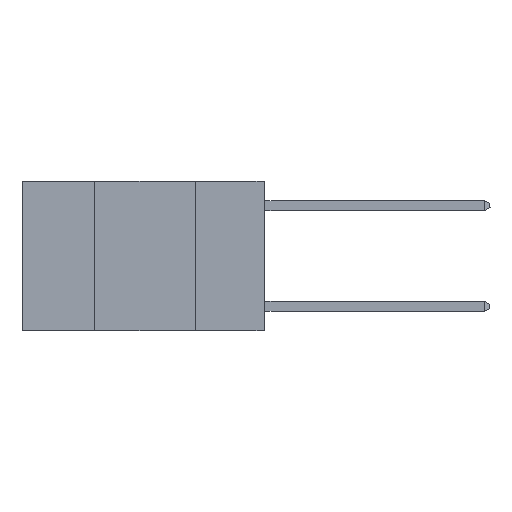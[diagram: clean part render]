
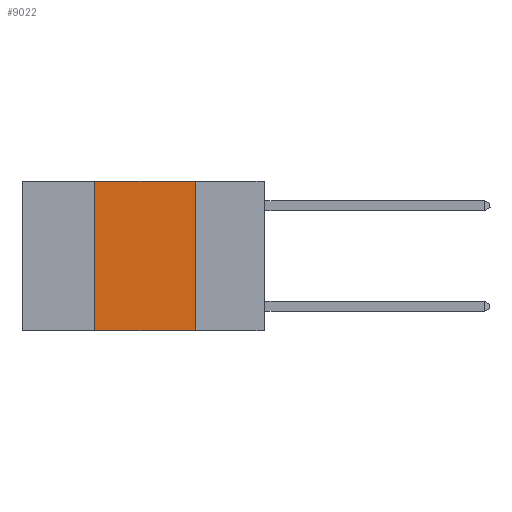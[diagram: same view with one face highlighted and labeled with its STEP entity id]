
A CAD part, left-side view. The second image highlights one B-rep face of the part: STEP entity #9022.
In plain terms, the highlighted planar face has unit normal (-1, 0, 0).
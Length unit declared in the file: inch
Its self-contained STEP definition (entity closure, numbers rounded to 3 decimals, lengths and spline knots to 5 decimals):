
#333 = CARTESIAN_POINT ( 'NONE',  ( 0., 0.17, -0.37 ) ) ;
#363 = ORIENTED_EDGE ( 'NONE', *, *, #10234, .F. ) ;
#574 = EDGE_LOOP ( 'NONE', ( #363, #10213, #7050, #12635 ) ) ;
#619 = VECTOR ( 'NONE', #13344, 39.37008 ) ;
#1965 = DIRECTION ( 'NONE',  ( 0., 0., 1. ) ) ;
#2409 = CARTESIAN_POINT ( 'NONE',  ( 0., 0.6, 0. ) ) ;
#2522 = VERTEX_POINT ( 'NONE', #14680 ) ;
#2852 = EDGE_CURVE ( 'NONE', #5796, #2522, #13362, .T. ) ;
#3385 = DIRECTION ( 'NONE',  ( 0., -1., 0. ) ) ;
#4080 = VECTOR ( 'NONE', #1965, 39.37008 ) ;
#4568 = CARTESIAN_POINT ( 'NONE',  ( 0., 0.42, -0.37 ) ) ;
#4858 = CARTESIAN_POINT ( 'NONE',  ( 0., 0.17, 0. ) ) ;
#5771 = DIRECTION ( 'NONE',  ( 0., -1., 0. ) ) ;
#5796 = VERTEX_POINT ( 'NONE', #4568 ) ;
#7012 = CARTESIAN_POINT ( 'NONE',  ( 0., 0.6, 0. ) ) ;
#7050 = ORIENTED_EDGE ( 'NONE', *, *, #2852, .F. ) ;
#7254 = DIRECTION ( 'NONE',  ( 1., 0., 0. ) ) ;
#7894 = AXIS2_PLACEMENT_3D ( 'NONE', #2409, #7254, #11761 ) ;
#8604 = VECTOR ( 'NONE', #5771, 39.37008 ) ;
#9022 = ADVANCED_FACE ( 'NONE', ( #11317 ), #14506, .F. ) ;
#9568 = VECTOR ( 'NONE', #3385, 39.37008 ) ;
#10213 = ORIENTED_EDGE ( 'NONE', *, *, #10775, .F. ) ;
#10234 = EDGE_CURVE ( 'NONE', #11382, #14653, #13172, .T. ) ;
#10775 = EDGE_CURVE ( 'NONE', #2522, #11382, #12385, .T. ) ;
#11046 = EDGE_CURVE ( 'NONE', #5796, #14653, #11806, .T. ) ;
#11317 = FACE_OUTER_BOUND ( 'NONE', #574, .T. ) ;
#11382 = VERTEX_POINT ( 'NONE', #13656 ) ;
#11761 = DIRECTION ( 'NONE',  ( 0., 0., -1. ) ) ;
#11806 = LINE ( 'NONE', #15409, #8604 ) ;
#12385 = LINE ( 'NONE', #7012, #9568 ) ;
#12635 = ORIENTED_EDGE ( 'NONE', *, *, #11046, .T. ) ;
#12897 = CARTESIAN_POINT ( 'NONE',  ( 0., 0.42, 0. ) ) ;
#13172 = LINE ( 'NONE', #4858, #619 ) ;
#13344 = DIRECTION ( 'NONE',  ( 0., 0., -1. ) ) ;
#13362 = LINE ( 'NONE', #12897, #4080 ) ;
#13656 = CARTESIAN_POINT ( 'NONE',  ( 0., 0.17, 0. ) ) ;
#14506 = PLANE ( 'NONE',  #7894 ) ;
#14653 = VERTEX_POINT ( 'NONE', #333 ) ;
#14680 = CARTESIAN_POINT ( 'NONE',  ( 0., 0.42, 0. ) ) ;
#15409 = CARTESIAN_POINT ( 'NONE',  ( 0., 0.6, -0.37 ) ) ;
